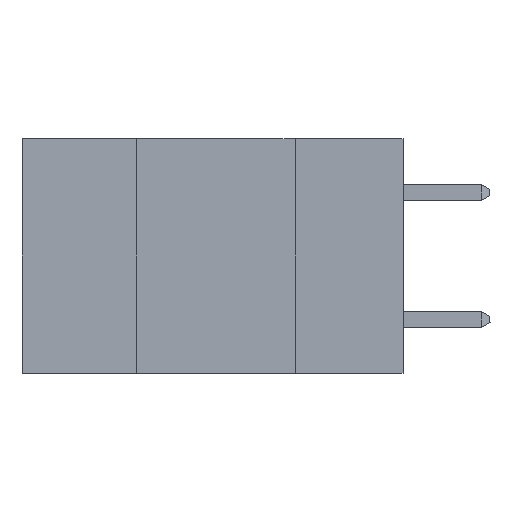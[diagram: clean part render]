
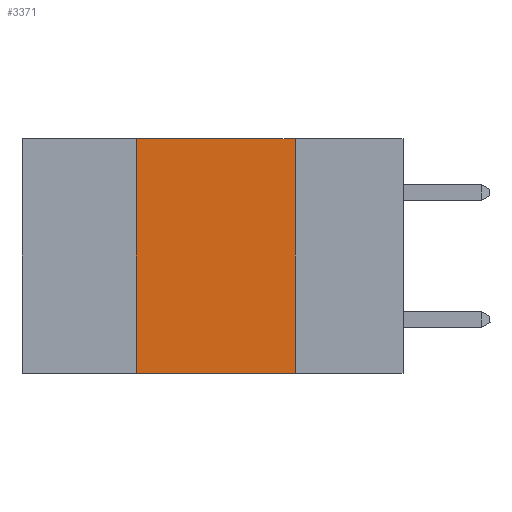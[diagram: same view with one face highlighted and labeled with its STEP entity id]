
A CAD part, left-side view. The second image highlights one B-rep face of the part: STEP entity #3371.
In plain terms, the highlighted planar face has unit normal (-1, 0, 0).
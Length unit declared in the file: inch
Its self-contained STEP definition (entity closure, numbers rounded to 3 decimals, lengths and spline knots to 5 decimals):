
#1139 = VERTEX_POINT ( 'NONE', #9439 ) ;
#2286 = ORIENTED_EDGE ( 'NONE', *, *, #12268, .F. ) ;
#3371 = ADVANCED_FACE ( 'NONE', ( #11301 ), #4013, .F. ) ;
#3919 = DIRECTION ( 'NONE',  ( 0., 0., -1. ) ) ;
#4013 = PLANE ( 'NONE',  #22728 ) ;
#4087 = VECTOR ( 'NONE', #8908, 39.37008 ) ;
#5122 = EDGE_CURVE ( 'NONE', #1139, #14458, #25989, .T. ) ;
#5918 = CARTESIAN_POINT ( 'NONE',  ( 0., 0.17, -0.37 ) ) ;
#7150 = CARTESIAN_POINT ( 'NONE',  ( 0., 0.17, 0. ) ) ;
#7964 = DIRECTION ( 'NONE',  ( 0., 0., 1. ) ) ;
#8067 = DIRECTION ( 'NONE',  ( 1., 0., 0. ) ) ;
#8908 = DIRECTION ( 'NONE',  ( 0., 0., -1. ) ) ;
#9396 = VERTEX_POINT ( 'NONE', #5918 ) ;
#9439 = CARTESIAN_POINT ( 'NONE',  ( 0., 0.42, -0.37 ) ) ;
#10303 = EDGE_CURVE ( 'NONE', #1139, #9396, #12608, .T. ) ;
#11301 = FACE_OUTER_BOUND ( 'NONE', #14838, .T. ) ;
#12268 = EDGE_CURVE ( 'NONE', #14458, #12623, #19843, .T. ) ;
#12608 = LINE ( 'NONE', #24870, #19017 ) ;
#12623 = VERTEX_POINT ( 'NONE', #7150 ) ;
#13225 = ORIENTED_EDGE ( 'NONE', *, *, #5122, .F. ) ;
#14442 = VECTOR ( 'NONE', #7964, 39.37008 ) ;
#14458 = VERTEX_POINT ( 'NONE', #17587 ) ;
#14838 = EDGE_LOOP ( 'NONE', ( #22938, #2286, #13225, #17740 ) ) ;
#17587 = CARTESIAN_POINT ( 'NONE',  ( 0., 0.42, 0. ) ) ;
#17740 = ORIENTED_EDGE ( 'NONE', *, *, #10303, .T. ) ;
#19017 = VECTOR ( 'NONE', #23061, 39.37008 ) ;
#19144 = CARTESIAN_POINT ( 'NONE',  ( 0., 0.17, 0. ) ) ;
#19505 = VECTOR ( 'NONE', #24493, 39.37008 ) ;
#19843 = LINE ( 'NONE', #25355, #19505 ) ;
#20174 = EDGE_CURVE ( 'NONE', #12623, #9396, #21121, .T. ) ;
#20543 = CARTESIAN_POINT ( 'NONE',  ( 0., 0.6, 0. ) ) ;
#21121 = LINE ( 'NONE', #19144, #4087 ) ;
#22728 = AXIS2_PLACEMENT_3D ( 'NONE', #20543, #8067, #3919 ) ;
#22938 = ORIENTED_EDGE ( 'NONE', *, *, #20174, .F. ) ;
#23061 = DIRECTION ( 'NONE',  ( 0., -1., 0. ) ) ;
#24493 = DIRECTION ( 'NONE',  ( 0., -1., 0. ) ) ;
#24560 = CARTESIAN_POINT ( 'NONE',  ( 0., 0.42, 0. ) ) ;
#24870 = CARTESIAN_POINT ( 'NONE',  ( 0., 0.6, -0.37 ) ) ;
#25355 = CARTESIAN_POINT ( 'NONE',  ( 0., 0.6, 0. ) ) ;
#25989 = LINE ( 'NONE', #24560, #14442 ) ;
